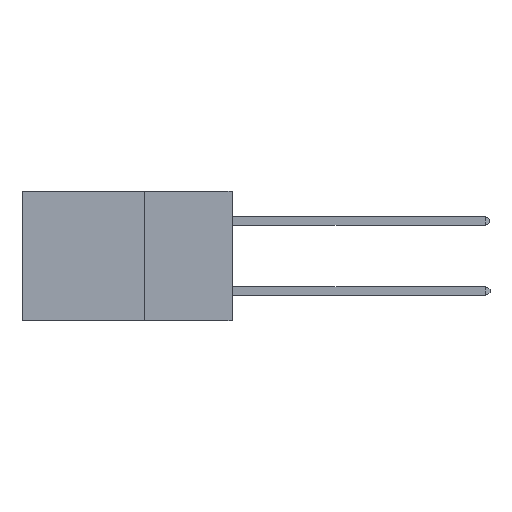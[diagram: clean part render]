
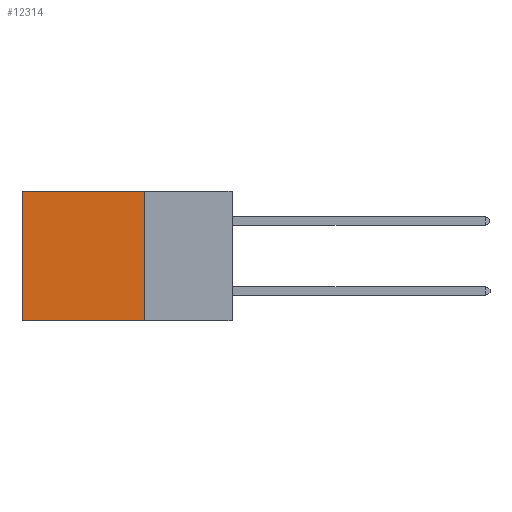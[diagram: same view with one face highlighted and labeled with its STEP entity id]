
A CAD part, left-side view. The second image highlights one B-rep face of the part: STEP entity #12314.
In plain terms, the highlighted planar face has unit normal (-1, 0, 0).
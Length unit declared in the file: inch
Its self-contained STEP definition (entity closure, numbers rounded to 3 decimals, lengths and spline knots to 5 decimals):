
#516 = CARTESIAN_POINT ( 'NONE',  ( 0.2875, 0.25, 0. ) ) ;
#963 = VECTOR ( 'NONE', #7411, 39.37008 ) ;
#1070 = ORIENTED_EDGE ( 'NONE', *, *, #3904, .T. ) ;
#1725 = DIRECTION ( 'NONE',  ( 0., 1., 0. ) ) ;
#2256 = DIRECTION ( 'NONE',  ( 1., 0., 0. ) ) ;
#3027 = CARTESIAN_POINT ( 'NONE',  ( 0.2875, 0.25, 0. ) ) ;
#3904 = EDGE_CURVE ( 'NONE', #19766, #9487, #10062, .T. ) ;
#4169 = VERTEX_POINT ( 'NONE', #18074 ) ;
#5704 = CARTESIAN_POINT ( 'NONE',  ( 0.2875, 0.25, 0. ) ) ;
#6119 = EDGE_CURVE ( 'NONE', #19766, #8786, #8934, .T. ) ;
#7411 = DIRECTION ( 'NONE',  ( 0., 1., 0. ) ) ;
#7499 = CARTESIAN_POINT ( 'NONE',  ( 0.2875, 0.25, -0.37 ) ) ;
#8025 = VECTOR ( 'NONE', #18237, 39.37008 ) ;
#8386 = CARTESIAN_POINT ( 'NONE',  ( 0.2875, 0.6, 0. ) ) ;
#8786 = VERTEX_POINT ( 'NONE', #7499 ) ;
#8934 = LINE ( 'NONE', #19574, #21485 ) ;
#9065 = PLANE ( 'NONE',  #12923 ) ;
#9079 = ORIENTED_EDGE ( 'NONE', *, *, #10935, .F. ) ;
#9487 = VERTEX_POINT ( 'NONE', #10786 ) ;
#10062 = LINE ( 'NONE', #5704, #963 ) ;
#10786 = CARTESIAN_POINT ( 'NONE',  ( 0.2875, 0.6, 0. ) ) ;
#10872 = EDGE_CURVE ( 'NONE', #9487, #4169, #20610, .T. ) ;
#10935 = EDGE_CURVE ( 'NONE', #8786, #4169, #19079, .T. ) ;
#11444 = DIRECTION ( 'NONE',  ( 0., 0., -1. ) ) ;
#12314 = ADVANCED_FACE ( 'NONE', ( #16464 ), #9065, .F. ) ;
#12923 = AXIS2_PLACEMENT_3D ( 'NONE', #516, #2256, #14071 ) ;
#14071 = DIRECTION ( 'NONE',  ( 0., 0., -1. ) ) ;
#14770 = VECTOR ( 'NONE', #1725, 39.37008 ) ;
#16464 = FACE_OUTER_BOUND ( 'NONE', #21095, .T. ) ;
#17445 = ORIENTED_EDGE ( 'NONE', *, *, #6119, .F. ) ;
#18074 = CARTESIAN_POINT ( 'NONE',  ( 0.2875, 0.6, -0.37 ) ) ;
#18237 = DIRECTION ( 'NONE',  ( 0., 0., -1. ) ) ;
#19079 = LINE ( 'NONE', #20003, #14770 ) ;
#19574 = CARTESIAN_POINT ( 'NONE',  ( 0.2875, 0.25, 0. ) ) ;
#19611 = ORIENTED_EDGE ( 'NONE', *, *, #10872, .T. ) ;
#19766 = VERTEX_POINT ( 'NONE', #3027 ) ;
#20003 = CARTESIAN_POINT ( 'NONE',  ( 0.2875, 0.25, -0.37 ) ) ;
#20610 = LINE ( 'NONE', #8386, #8025 ) ;
#21095 = EDGE_LOOP ( 'NONE', ( #19611, #9079, #17445, #1070 ) ) ;
#21485 = VECTOR ( 'NONE', #11444, 39.37008 ) ;
